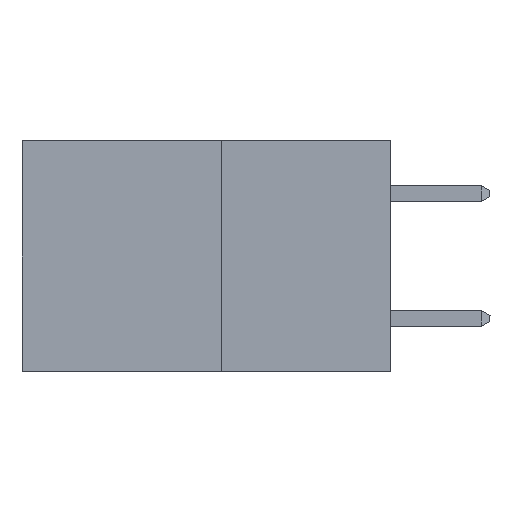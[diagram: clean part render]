
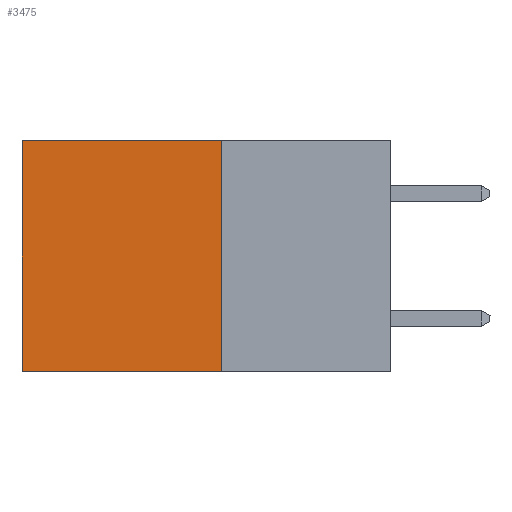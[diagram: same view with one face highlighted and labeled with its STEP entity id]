
A CAD part, left-side view. The second image highlights one B-rep face of the part: STEP entity #3475.
In plain terms, the highlighted planar face has unit normal (-1, 0, 0).
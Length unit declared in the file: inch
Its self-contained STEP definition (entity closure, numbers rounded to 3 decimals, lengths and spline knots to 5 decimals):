
#935 = CARTESIAN_POINT ( 'NONE',  ( 0.277, 0.27, 0. ) ) ;
#2697 = DIRECTION ( 'NONE',  ( 0., 0., -1. ) ) ;
#3260 = VECTOR ( 'NONE', #10304, 39.37008 ) ;
#3350 = EDGE_CURVE ( 'NONE', #20978, #14512, #14635, .T. ) ;
#3475 = ADVANCED_FACE ( 'NONE', ( #4439 ), #26961, .F. ) ;
#3840 = VECTOR ( 'NONE', #13667, 39.37008 ) ;
#4172 = CARTESIAN_POINT ( 'NONE',  ( 0.277, 0.59, 0. ) ) ;
#4439 = FACE_OUTER_BOUND ( 'NONE', #13796, .T. ) ;
#7799 = CARTESIAN_POINT ( 'NONE',  ( 0.277, 0.27, -0.37 ) ) ;
#10304 = DIRECTION ( 'NONE',  ( 0., 1., 0. ) ) ;
#10975 = VERTEX_POINT ( 'NONE', #4172 ) ;
#11004 = CARTESIAN_POINT ( 'NONE',  ( 0.277, 0.59, -0.37 ) ) ;
#13667 = DIRECTION ( 'NONE',  ( 0., 0., -1. ) ) ;
#13796 = EDGE_LOOP ( 'NONE', ( #20223, #26139, #16095, #19602 ) ) ;
#14512 = VERTEX_POINT ( 'NONE', #11004 ) ;
#14635 = LINE ( 'NONE', #28473, #19493 ) ;
#16095 = ORIENTED_EDGE ( 'NONE', *, *, #23068, .F. ) ;
#17113 = CARTESIAN_POINT ( 'NONE',  ( 0.277, 0.27, -0.37 ) ) ;
#17393 = LINE ( 'NONE', #18582, #3840 ) ;
#18582 = CARTESIAN_POINT ( 'NONE',  ( 0.277, 0.59, -0.37 ) ) ;
#19493 = VECTOR ( 'NONE', #28433, 39.37008 ) ;
#19602 = ORIENTED_EDGE ( 'NONE', *, *, #23177, .T. ) ;
#20223 = ORIENTED_EDGE ( 'NONE', *, *, #30409, .T. ) ;
#20978 = VERTEX_POINT ( 'NONE', #7799 ) ;
#23068 = EDGE_CURVE ( 'NONE', #26229, #20978, #24770, .T. ) ;
#23177 = EDGE_CURVE ( 'NONE', #26229, #10975, #28131, .T. ) ;
#24696 = AXIS2_PLACEMENT_3D ( 'NONE', #25911, #25812, #25807 ) ;
#24770 = LINE ( 'NONE', #17113, #31118 ) ;
#25807 = DIRECTION ( 'NONE',  ( 0., 0., -1. ) ) ;
#25812 = DIRECTION ( 'NONE',  ( 1., 0., 0. ) ) ;
#25911 = CARTESIAN_POINT ( 'NONE',  ( 0.277, 0.27, -0.37 ) ) ;
#26139 = ORIENTED_EDGE ( 'NONE', *, *, #3350, .F. ) ;
#26229 = VERTEX_POINT ( 'NONE', #935 ) ;
#26961 = PLANE ( 'NONE',  #24696 ) ;
#27137 = CARTESIAN_POINT ( 'NONE',  ( 0.277, 0.27, 0. ) ) ;
#28131 = LINE ( 'NONE', #27137, #3260 ) ;
#28433 = DIRECTION ( 'NONE',  ( 0., 1., 0. ) ) ;
#28473 = CARTESIAN_POINT ( 'NONE',  ( 0.277, 0.27, -0.37 ) ) ;
#30409 = EDGE_CURVE ( 'NONE', #10975, #14512, #17393, .T. ) ;
#31118 = VECTOR ( 'NONE', #2697, 39.37008 ) ;
